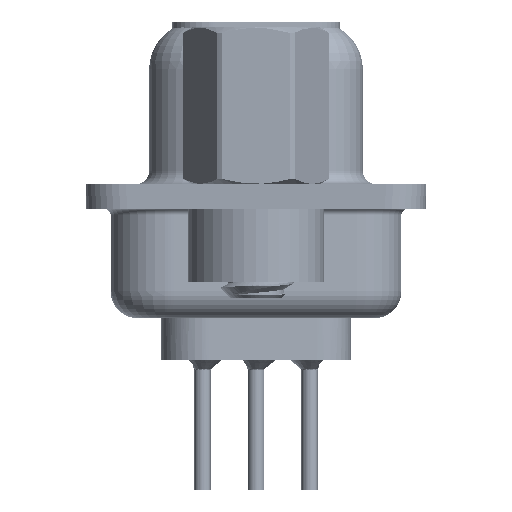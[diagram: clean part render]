
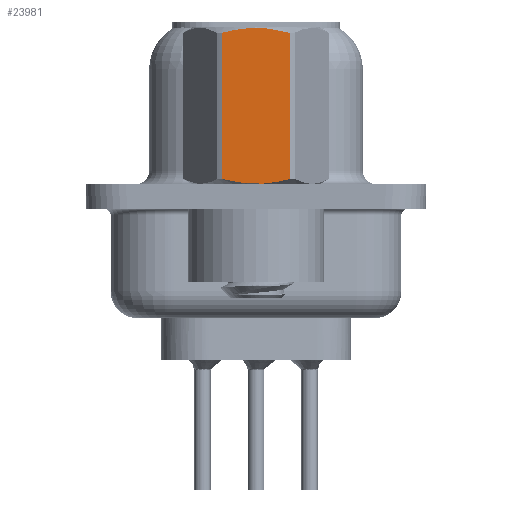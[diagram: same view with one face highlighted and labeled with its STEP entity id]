
A CAD part, left-side view. The second image highlights one B-rep face of the part: STEP entity #23981.
In plain terms, the highlighted planar face has unit normal (-1, 0, 0).
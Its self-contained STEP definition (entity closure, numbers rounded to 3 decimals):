
#1630 = CARTESIAN_POINT ( 'NONE',  ( -2.381, 0.215, 6.232 ) ) ;
#2291 = EDGE_CURVE ( 'NONE', #26152, #12478, #36340, .T. ) ;
#2420 = ORIENTED_EDGE ( 'NONE', *, *, #24348, .T. ) ;
#3014 = CARTESIAN_POINT ( 'NONE',  ( -2.381, -1.273, 6.048 ) ) ;
#3055 = CARTESIAN_POINT ( 'NONE',  ( -2.381, 0.215, 0.468 ) ) ;
#5241 = DIRECTION ( 'NONE',  ( 0., 0., 1. ) ) ;
#6221 = LINE ( 'NONE', #20102, #18907 ) ;
#7398 = EDGE_LOOP ( 'NONE', ( #2420, #31036, #34505, #21916 ) ) ;
#8255 = CARTESIAN_POINT ( 'NONE',  ( -2.381, -1.066, 0.596 ) ) ;
#8440 = CARTESIAN_POINT ( 'NONE',  ( -2.381, -1.273, 6.048 ) ) ;
#8673 = CARTESIAN_POINT ( 'NONE',  ( -2.381, -1.066, 6.104 ) ) ;
#8990 = DIRECTION ( 'NONE',  ( -1., 0., 0. ) ) ;
#12478 = VERTEX_POINT ( 'NONE', #3014 ) ;
#14394 = CARTESIAN_POINT ( 'NONE',  ( -2.381, 1.273, 6.048 ) ) ;
#14637 = CARTESIAN_POINT ( 'NONE',  ( -2.381, -0.215, 0.468 ) ) ;
#14704 = VERTEX_POINT ( 'NONE', #19297 ) ;
#15048 = CARTESIAN_POINT ( 'NONE',  ( -2.381, 0.428, 6.215 ) ) ;
#17119 = CARTESIAN_POINT ( 'NONE',  ( -2.381, 1.375, -3.75 ) ) ;
#18876 = CARTESIAN_POINT ( 'NONE',  ( -2.381, -0.432, 6.215 ) ) ;
#18907 = VECTOR ( 'NONE', #33916, 1000. ) ;
#18912 = CARTESIAN_POINT ( 'NONE',  ( -2.381, -1.273, 0.652 ) ) ;
#19297 = CARTESIAN_POINT ( 'NONE',  ( -2.381, 1.273, 0.652 ) ) ;
#19337 = CARTESIAN_POINT ( 'NONE',  ( -2.381, 1.065, 6.104 ) ) ;
#20102 = CARTESIAN_POINT ( 'NONE',  ( -2.381, 1.273, 3.792 ) ) ;
#21234 = CARTESIAN_POINT ( 'NONE',  ( -2.381, 1.273, 0.652 ) ) ;
#21270 = EDGE_CURVE ( 'NONE', #12478, #39986, #39428, .T. ) ;
#21916 = ORIENTED_EDGE ( 'NONE', *, *, #28555, .T. ) ;
#22296 = CARTESIAN_POINT ( 'NONE',  ( -2.381, -0.858, 6.15 ) ) ;
#23056 = VECTOR ( 'NONE', #5241, 1000. ) ;
#23747 = CARTESIAN_POINT ( 'NONE',  ( -2.381, 1.065, 0.596 ) ) ;
#23981 = ADVANCED_FACE ( 'NONE', ( #36662 ), #44756, .T. ) ;
#24348 = EDGE_CURVE ( 'NONE', #14704, #26152, #40824, .T. ) ;
#25904 = CARTESIAN_POINT ( 'NONE',  ( -2.381, -1.273, 0.652 ) ) ;
#26152 = VERTEX_POINT ( 'NONE', #25904 ) ;
#28555 = EDGE_CURVE ( 'NONE', #39986, #14704, #6221, .T. ) ;
#28874 = CARTESIAN_POINT ( 'NONE',  ( -2.381, -1.273, 3.792 ) ) ;
#31036 = ORIENTED_EDGE ( 'NONE', *, *, #2291, .T. ) ;
#33141 = CARTESIAN_POINT ( 'NONE',  ( -2.381, 1.273, 6.048 ) ) ;
#33916 = DIRECTION ( 'NONE',  ( 0., 0., -1. ) ) ;
#34135 = CARTESIAN_POINT ( 'NONE',  ( -2.381, 0.428, 0.485 ) ) ;
#34505 = ORIENTED_EDGE ( 'NONE', *, *, #21270, .T. ) ;
#35340 = AXIS2_PLACEMENT_3D ( 'NONE', #17119, #8990, #44516 ) ;
#35918 = CARTESIAN_POINT ( 'NONE',  ( -2.381, -0.858, 0.55 ) ) ;
#36325 = CARTESIAN_POINT ( 'NONE',  ( -2.381, -0.215, 6.232 ) ) ;
#36340 = LINE ( 'NONE', #28874, #23056 ) ;
#36662 = FACE_OUTER_BOUND ( 'NONE', #7398, .T. ) ;
#37547 = CARTESIAN_POINT ( 'NONE',  ( -2.381, 0.853, 0.549 ) ) ;
#39428 = B_SPLINE_CURVE_WITH_KNOTS ( 'NONE', 3,
 ( #8440, #8673, #22296, #18876, #36325, #1630, #15048, #39940, #19337, #33141 ),
 .UNSPECIFIED., .F., .F.,
 ( 4, 2, 2, 2, 4 ),
 ( 0.001, 0.002, 0.002, 0.003, 0.004 ),
 .UNSPECIFIED. ) ;
#39940 = CARTESIAN_POINT ( 'NONE',  ( -2.381, 0.853, 6.151 ) ) ;
#39986 = VERTEX_POINT ( 'NONE', #14394 ) ;
#40824 = B_SPLINE_CURVE_WITH_KNOTS ( 'NONE', 3,
 ( #21234, #23747, #37547, #34135, #3055, #14637, #42489, #35918, #8255, #18912 ),
 .UNSPECIFIED., .F., .F.,
 ( 4, 2, 2, 2, 4 ),
 ( 0.003, 0.003, 0.004, 0.004, 0.005 ),
 .UNSPECIFIED. ) ;
#42489 = CARTESIAN_POINT ( 'NONE',  ( -2.381, -0.432, 0.485 ) ) ;
#44516 = DIRECTION ( 'NONE',  ( 0., -1., 0. ) ) ;
#44756 = PLANE ( 'NONE',  #35340 ) ;
